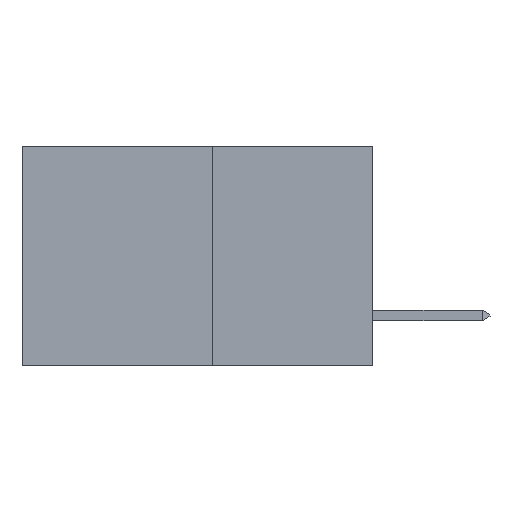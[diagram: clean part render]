
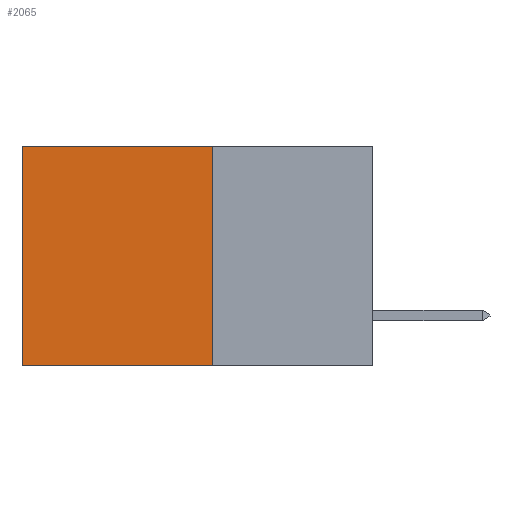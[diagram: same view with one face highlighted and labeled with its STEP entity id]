
A CAD part, left-side view. The second image highlights one B-rep face of the part: STEP entity #2065.
In plain terms, the highlighted planar face has unit normal (-1, 0, 0).
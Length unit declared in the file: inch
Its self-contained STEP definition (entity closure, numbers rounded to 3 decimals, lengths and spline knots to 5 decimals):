
#183 = VERTEX_POINT ( 'NONE', #6877 ) ;
#210 = CARTESIAN_POINT ( 'NONE',  ( 0.277, 0.27, 0. ) ) ;
#996 = DIRECTION ( 'NONE',  ( 1., 0., 0. ) ) ;
#1153 = FACE_OUTER_BOUND ( 'NONE', #2476, .T. ) ;
#1190 = ORIENTED_EDGE ( 'NONE', *, *, #1439, .T. ) ;
#1418 = CARTESIAN_POINT ( 'NONE',  ( 0.277, 0.27, -0.37 ) ) ;
#1439 = EDGE_CURVE ( 'NONE', #6957, #10004, #6223, .T. ) ;
#1634 = VECTOR ( 'NONE', #5421, 39.37008 ) ;
#1721 = ORIENTED_EDGE ( 'NONE', *, *, #8556, .T. ) ;
#1860 = LINE ( 'NONE', #3557, #6112 ) ;
#2065 = ADVANCED_FACE ( 'NONE', ( #1153 ), #2892, .F. ) ;
#2240 = VECTOR ( 'NONE', #2877, 39.37008 ) ;
#2396 = CARTESIAN_POINT ( 'NONE',  ( 0.277, 0.27, 0. ) ) ;
#2406 = VECTOR ( 'NONE', #3377, 39.37008 ) ;
#2476 = EDGE_LOOP ( 'NONE', ( #1721, #2494, #2898, #1190 ) ) ;
#2494 = ORIENTED_EDGE ( 'NONE', *, *, #9747, .F. ) ;
#2704 = DIRECTION ( 'NONE',  ( 0., 0., -1. ) ) ;
#2877 = DIRECTION ( 'NONE',  ( 0., 1., 0. ) ) ;
#2892 = PLANE ( 'NONE',  #4730 ) ;
#2898 = ORIENTED_EDGE ( 'NONE', *, *, #7185, .F. ) ;
#3377 = DIRECTION ( 'NONE',  ( 0., 0., -1. ) ) ;
#3557 = CARTESIAN_POINT ( 'NONE',  ( 0.277, 0.27, -0.37 ) ) ;
#4730 = AXIS2_PLACEMENT_3D ( 'NONE', #1418, #996, #2704 ) ;
#4856 = LINE ( 'NONE', #9452, #2406 ) ;
#5421 = DIRECTION ( 'NONE',  ( 0., 0., -1. ) ) ;
#6112 = VECTOR ( 'NONE', #7464, 39.37008 ) ;
#6176 = CARTESIAN_POINT ( 'NONE',  ( 0.277, 0.27, -0.37 ) ) ;
#6223 = LINE ( 'NONE', #2396, #2240 ) ;
#6877 = CARTESIAN_POINT ( 'NONE',  ( 0.277, 0.59, -0.37 ) ) ;
#6957 = VERTEX_POINT ( 'NONE', #210 ) ;
#7017 = CARTESIAN_POINT ( 'NONE',  ( 0.277, 0.59, 0. ) ) ;
#7185 = EDGE_CURVE ( 'NONE', #6957, #9990, #7957, .T. ) ;
#7464 = DIRECTION ( 'NONE',  ( 0., 1., 0. ) ) ;
#7741 = CARTESIAN_POINT ( 'NONE',  ( 0.277, 0.27, -0.37 ) ) ;
#7957 = LINE ( 'NONE', #6176, #1634 ) ;
#8556 = EDGE_CURVE ( 'NONE', #10004, #183, #4856, .T. ) ;
#9452 = CARTESIAN_POINT ( 'NONE',  ( 0.277, 0.59, -0.37 ) ) ;
#9747 = EDGE_CURVE ( 'NONE', #9990, #183, #1860, .T. ) ;
#9990 = VERTEX_POINT ( 'NONE', #7741 ) ;
#10004 = VERTEX_POINT ( 'NONE', #7017 ) ;
